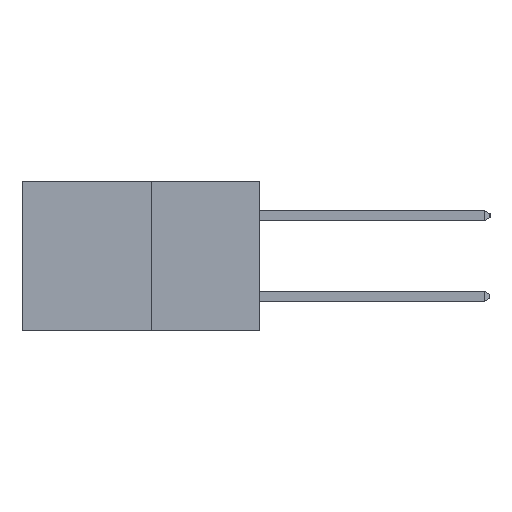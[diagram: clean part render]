
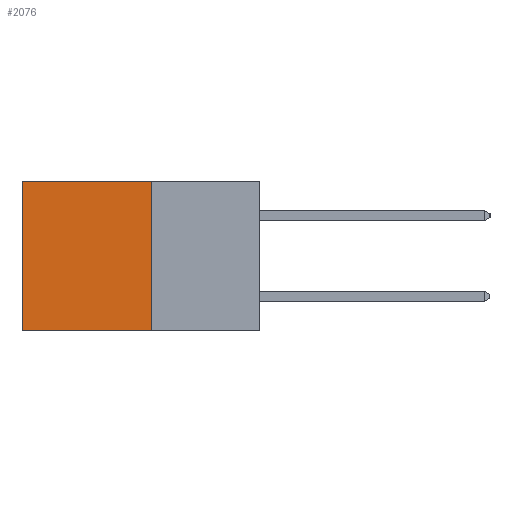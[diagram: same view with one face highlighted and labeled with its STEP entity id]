
A CAD part, left-side view. The second image highlights one B-rep face of the part: STEP entity #2076.
In plain terms, the highlighted planar face has unit normal (-1, 0, 0).
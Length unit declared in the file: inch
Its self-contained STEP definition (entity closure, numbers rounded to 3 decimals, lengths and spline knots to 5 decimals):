
#617 = CARTESIAN_POINT ( 'NONE',  ( 0.277, 0.59, 0. ) ) ;
#1322 = EDGE_CURVE ( 'NONE', #9192, #11834, #2495, .T. ) ;
#1390 = VECTOR ( 'NONE', #8816, 39.37008 ) ;
#1393 = VERTEX_POINT ( 'NONE', #617 ) ;
#1426 = CARTESIAN_POINT ( 'NONE',  ( 0.277, 0.27, -0.37 ) ) ;
#1522 = CARTESIAN_POINT ( 'NONE',  ( 0.277, 0.27, 0. ) ) ;
#1626 = DIRECTION ( 'NONE',  ( 0., 1., 0. ) ) ;
#1746 = CARTESIAN_POINT ( 'NONE',  ( 0.277, 0.27, -0.37 ) ) ;
#2015 = CARTESIAN_POINT ( 'NONE',  ( 0.277, 0.27, -0.37 ) ) ;
#2076 = ADVANCED_FACE ( 'NONE', ( #11617 ), #4330, .F. ) ;
#2495 = LINE ( 'NONE', #2015, #12681 ) ;
#2865 = VECTOR ( 'NONE', #1626, 39.37008 ) ;
#2888 = CARTESIAN_POINT ( 'NONE',  ( 0.277, 0.59, -0.37 ) ) ;
#4330 = PLANE ( 'NONE',  #9989 ) ;
#4424 = ORIENTED_EDGE ( 'NONE', *, *, #6235, .T. ) ;
#5634 = EDGE_CURVE ( 'NONE', #9212, #1393, #8153, .T. ) ;
#6235 = EDGE_CURVE ( 'NONE', #1393, #11834, #12403, .T. ) ;
#6979 = ORIENTED_EDGE ( 'NONE', *, *, #1322, .F. ) ;
#8153 = LINE ( 'NONE', #1522, #2865 ) ;
#8204 = ORIENTED_EDGE ( 'NONE', *, *, #5634, .T. ) ;
#8816 = DIRECTION ( 'NONE',  ( 0., 0., -1. ) ) ;
#9192 = VERTEX_POINT ( 'NONE', #1426 ) ;
#9212 = VERTEX_POINT ( 'NONE', #11455 ) ;
#9448 = EDGE_CURVE ( 'NONE', #9212, #9192, #12014, .T. ) ;
#9687 = EDGE_LOOP ( 'NONE', ( #4424, #6979, #9889, #8204 ) ) ;
#9833 = VECTOR ( 'NONE', #11994, 39.37008 ) ;
#9876 = DIRECTION ( 'NONE',  ( 0., 1., 0. ) ) ;
#9889 = ORIENTED_EDGE ( 'NONE', *, *, #9448, .F. ) ;
#9989 = AXIS2_PLACEMENT_3D ( 'NONE', #13022, #12541, #12698 ) ;
#10999 = CARTESIAN_POINT ( 'NONE',  ( 0.277, 0.59, -0.37 ) ) ;
#11455 = CARTESIAN_POINT ( 'NONE',  ( 0.277, 0.27, 0. ) ) ;
#11617 = FACE_OUTER_BOUND ( 'NONE', #9687, .T. ) ;
#11834 = VERTEX_POINT ( 'NONE', #2888 ) ;
#11994 = DIRECTION ( 'NONE',  ( 0., 0., -1. ) ) ;
#12014 = LINE ( 'NONE', #1746, #1390 ) ;
#12403 = LINE ( 'NONE', #10999, #9833 ) ;
#12541 = DIRECTION ( 'NONE',  ( 1., 0., 0. ) ) ;
#12681 = VECTOR ( 'NONE', #9876, 39.37008 ) ;
#12698 = DIRECTION ( 'NONE',  ( 0., 0., -1. ) ) ;
#13022 = CARTESIAN_POINT ( 'NONE',  ( 0.277, 0.27, -0.37 ) ) ;
